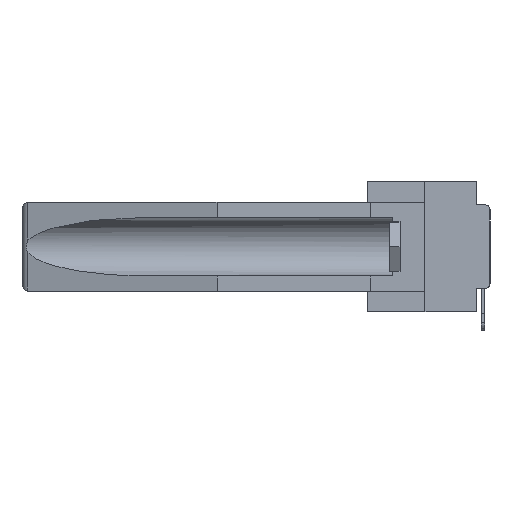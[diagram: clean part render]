
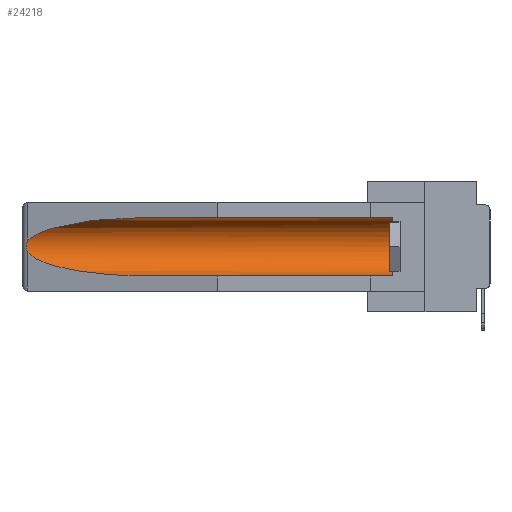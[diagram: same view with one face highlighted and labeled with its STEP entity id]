
A CAD part, left-side view. The second image highlights one B-rep face of the part: STEP entity #24218.
In plain terms, the highlighted cylindrical face has radius 2.857 mm (diameter 5.715 mm), a partial arc.
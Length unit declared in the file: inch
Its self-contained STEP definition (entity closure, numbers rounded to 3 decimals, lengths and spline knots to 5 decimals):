
#1475 = CARTESIAN_POINT ( 'NONE',  ( 0.26537, 1.52718, -0.14972 ) ) ;
#1729 = ORIENTED_EDGE ( 'NONE', *, *, #2618, .T. ) ;
#2052 = CARTESIAN_POINT ( 'NONE',  ( 0.26537, 1.52718, -0.14972 ) ) ;
#2618 = EDGE_CURVE ( 'NONE', #25198, #7295, #24206, .T. ) ;
#2832 = AXIS2_PLACEMENT_3D ( 'NONE', #10856, #16551, #18814 ) ;
#3126 = LINE ( 'NONE', #13038, #8567 ) ;
#3227 = FACE_OUTER_BOUND ( 'NONE', #23790, .T. ) ;
#3811 = EDGE_CURVE ( 'NONE', #13565, #25198, #22959, .T. ) ;
#3816 = CARTESIAN_POINT ( 'NONE',  ( 0.26537, 1.52718, -0.14972 ) ) ;
#3856 = ORIENTED_EDGE ( 'NONE', *, *, #8971, .T. ) ;
#3986 = CARTESIAN_POINT ( 'NONE',  ( 0.26537, 1.52718, -0.19328 ) ) ;
#4495 = CARTESIAN_POINT ( 'NONE',  ( 0.21114, 1.30732, -0.284 ) ) ;
#5933 = DIRECTION ( 'NONE',  ( 0., 1., 0. ) ) ;
#6681 = CARTESIAN_POINT ( 'NONE',  ( 0.25451, 1.48313, -0.09465 ) ) ;
#7295 = VERTEX_POINT ( 'NONE', #24707 ) ;
#7301 = ORIENTED_EDGE ( 'NONE', *, *, #32600, .T. ) ;
#8436 = CARTESIAN_POINT ( 'NONE',  ( 0.155, -0.30754, -0.1715 ) ) ;
#8567 = VECTOR ( 'NONE', #31925, 39.37008 ) ;
#8880 = VERTEX_POINT ( 'NONE', #24199 ) ;
#8971 = EDGE_CURVE ( 'NONE', #27457, #8880, #31054, .T. ) ;
#9223 = CARTESIAN_POINT ( 'NONE',  ( 0.2675, 1.53308, -0.17534 ) ) ;
#9724 = CARTESIAN_POINT ( 'NONE',  ( 0.155, 1.07973, -0.059 ) ) ;
#10064 = CARTESIAN_POINT ( 'NONE',  ( 0.25451, 1.48313, -0.24835 ) ) ;
#10856 = CARTESIAN_POINT ( 'NONE',  ( 0.155, 0.126, -0.1715 ) ) ;
#11148 = LINE ( 'NONE', #32637, #32829 ) ;
#11723 = CARTESIAN_POINT ( 'NONE',  ( 0.21114, 1.30732, -0.059 ) ) ;
#13038 = CARTESIAN_POINT ( 'NONE',  ( 0.155, -0.30754, -0.284 ) ) ;
#13565 = VERTEX_POINT ( 'NONE', #2052 ) ;
#13801 = DIRECTION ( 'NONE',  ( 0., 0., 1. ) ) ;
#14159 = DIRECTION ( 'NONE',  ( 0., 1., 0. ) ) ;
#14411 = CARTESIAN_POINT ( 'NONE',  ( 0.26597, 1.52961, -0.15275 ) ) ;
#14549 = EDGE_CURVE ( 'NONE', #8880, #31865, #11148, .T. ) ;
#14582 = CARTESIAN_POINT ( 'NONE',  ( 0.26537, 1.52718, -0.19328 ) ) ;
#16124 = EDGE_CURVE ( 'NONE', #27457, #7295, #3126, .T. ) ;
#16551 = DIRECTION ( 'NONE',  ( 0., -1., 0. ) ) ;
#17096 = CARTESIAN_POINT ( 'NONE',  ( 0.155, 1.07973, -0.059 ) ) ;
#17399 = ORIENTED_EDGE ( 'NONE', *, *, #3811, .T. ) ;
#18814 = DIRECTION ( 'NONE',  ( 0., 0., 1. ) ) ;
#19775 = CARTESIAN_POINT ( 'NONE',  ( 0.2673, 1.53269, -0.17917 ) ) ;
#20446 = CARTESIAN_POINT ( 'NONE',  ( 0.155, 1.07973, -0.284 ) ) ;
#21556 =( BOUNDED_CURVE ( )  B_SPLINE_CURVE ( 3, ( #17096, #11723, #6681, #1475 ),
 .UNSPECIFIED., .F., .F. ) 
 B_SPLINE_CURVE_WITH_KNOTS ( ( 4, 4 ),
 ( 4.71239, 6.08839 ),
 .UNSPECIFIED. ) 
 CURVE ( )  GEOMETRIC_REPRESENTATION_ITEM ( )  RATIONAL_B_SPLINE_CURVE ( ( 1., 0.848, 0.848, 1. ) ) 
 REPRESENTATION_ITEM ( '' )  );
#21772 = CYLINDRICAL_SURFACE ( 'NONE', #25273, 0.1125 ) ;
#22379 = CARTESIAN_POINT ( 'NONE',  ( 0.2673, 1.5327, -0.16383 ) ) ;
#22864 = ORIENTED_EDGE ( 'NONE', *, *, #16124, .F. ) ;
#22959 = B_SPLINE_CURVE_WITH_KNOTS ( 'NONE', 3,
 ( #3816, #14411, #24980, #22379, #32971, #9223, #19775, #27745, #30358, #14582 ),
 .UNSPECIFIED., .F., .F.,
 ( 4, 2, 2, 2, 4 ),
 ( 0., 0.00029, 0.00058, 0.00087, 0.00117 ),
 .UNSPECIFIED. ) ;
#23790 = EDGE_LOOP ( 'NONE', ( #7301, #17399, #1729, #22864, #3856, #30855 ) ) ;
#24199 = CARTESIAN_POINT ( 'NONE',  ( 0.155, 0.126, -0.059 ) ) ;
#24206 =( BOUNDED_CURVE ( )  B_SPLINE_CURVE ( 3, ( #3986, #10064, #4495, #20446 ),
 .UNSPECIFIED., .F., .F. ) 
 B_SPLINE_CURVE_WITH_KNOTS ( ( 4, 4 ),
 ( 0.1948, 1.5708 ),
 .UNSPECIFIED. ) 
 CURVE ( )  GEOMETRIC_REPRESENTATION_ITEM ( )  RATIONAL_B_SPLINE_CURVE ( ( 1., 0.848, 0.848, 1. ) ) 
 REPRESENTATION_ITEM ( '' )  );
#24218 = ADVANCED_FACE ( 'NONE', ( #3227 ), #21772, .F. ) ;
#24707 = CARTESIAN_POINT ( 'NONE',  ( 0.155, 1.07973, -0.284 ) ) ;
#24980 = CARTESIAN_POINT ( 'NONE',  ( 0.26654, 1.53092, -0.15636 ) ) ;
#25198 = VERTEX_POINT ( 'NONE', #29801 ) ;
#25273 = AXIS2_PLACEMENT_3D ( 'NONE', #8436, #14159, #13801 ) ;
#27457 = VERTEX_POINT ( 'NONE', #27465 ) ;
#27465 = CARTESIAN_POINT ( 'NONE',  ( 0.155, 0.126, -0.284 ) ) ;
#27745 = CARTESIAN_POINT ( 'NONE',  ( 0.26655, 1.53094, -0.18657 ) ) ;
#29801 = CARTESIAN_POINT ( 'NONE',  ( 0.26537, 1.52718, -0.19328 ) ) ;
#30358 = CARTESIAN_POINT ( 'NONE',  ( 0.26597, 1.5296, -0.19026 ) ) ;
#30855 = ORIENTED_EDGE ( 'NONE', *, *, #14549, .T. ) ;
#31054 = CIRCLE ( 'NONE', #2832, 0.1125 ) ;
#31865 = VERTEX_POINT ( 'NONE', #9724 ) ;
#31925 = DIRECTION ( 'NONE',  ( 0., 1., 0. ) ) ;
#32600 = EDGE_CURVE ( 'NONE', #31865, #13565, #21556, .T. ) ;
#32637 = CARTESIAN_POINT ( 'NONE',  ( 0.155, -0.30754, -0.059 ) ) ;
#32829 = VECTOR ( 'NONE', #5933, 39.37008 ) ;
#32971 = CARTESIAN_POINT ( 'NONE',  ( 0.2675, 1.53308, -0.16763 ) ) ;
